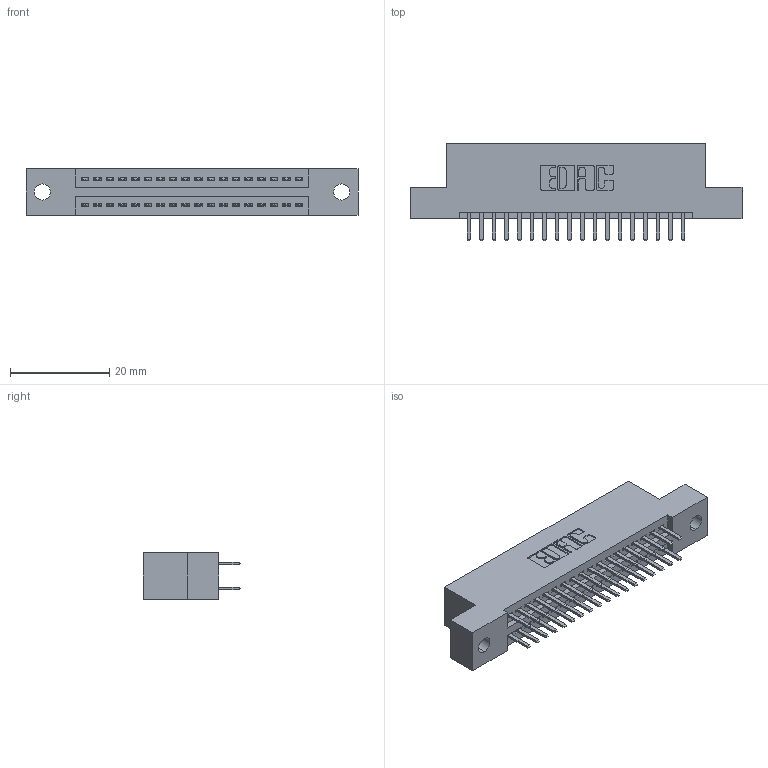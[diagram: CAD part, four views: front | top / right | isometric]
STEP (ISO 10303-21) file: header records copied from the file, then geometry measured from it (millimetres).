
FILE_DESCRIPTION (( 'STEP AP203' ), '1' );
FILE_NAME ('345-036-520-202.STEP', '2019-10-28T11:14:25', ( '' ), ( '' ), 'SwSTEP 2.0', 'SolidWorks 2016', '' );
FILE_SCHEMA (( 'CONFIG_CONTROL_DESIGN' ));
Length unit declared in the file: inch
Products named in the file (3): 345 Part_Flush Mounting Lugs - 0.128 Dia; 345-036-520-202; 345-292-001_345-293-120
Assembly tree (37 placements, depth 2):
  345-036-520-202
    345 Part_Flush Mounting Lugs - 0.128 Dia
    345-292-001_345-293-120  x36
Bounding box: 66.93 x 19.68 x 9.4 mm (x, y, z)
Volume: 6226.3 mm3; surface area: 8432.3 mm2
Topology: 37 solids, 37 shells, 2070 faces, 5993 edges, 3898 vertices
Faces by surface type: plane 1340, cylinder 730
Entity records: 17471 total; most frequent: CARTESIAN_POINT 2964, ORIENTED_EDGE 2886, DIRECTION 2631, EDGE_CURVE 1443, LINE 1235, VECTOR 1235, VERTEX_POINT 958, AXIS2_PLACEMENT_3D 698
